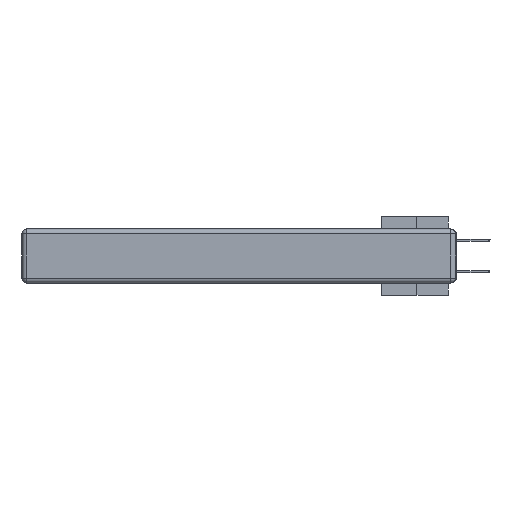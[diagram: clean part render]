
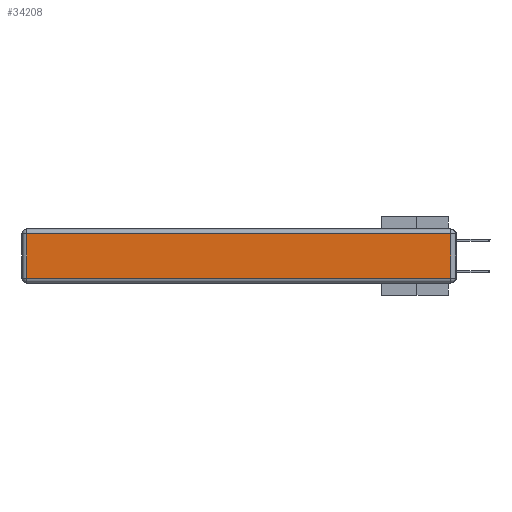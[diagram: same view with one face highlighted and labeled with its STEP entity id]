
A CAD part, left-side view. The second image highlights one B-rep face of the part: STEP entity #34208.
In plain terms, the highlighted planar face has unit normal (-1, 0, 0).
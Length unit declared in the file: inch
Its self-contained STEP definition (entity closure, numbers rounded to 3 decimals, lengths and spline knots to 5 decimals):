
#106 = CARTESIAN_POINT ( 'NONE',  ( 0., 0.03, -0.03 ) ) ;
#294 = CARTESIAN_POINT ( 'NONE',  ( 0., 2.72, -0.313 ) ) ;
#669 = VERTEX_POINT ( 'NONE', #106 ) ;
#1740 = DIRECTION ( 'NONE',  ( 0., -1., 0. ) ) ;
#2527 = DIRECTION ( 'NONE',  ( -1., 0., 0. ) ) ;
#2875 = VECTOR ( 'NONE', #11529, 39.37008 ) ;
#4321 = CARTESIAN_POINT ( 'NONE',  ( 0., 0.03, -0.313 ) ) ;
#6305 = ORIENTED_EDGE ( 'NONE', *, *, #15452, .T. ) ;
#6931 = EDGE_CURVE ( 'NONE', #669, #9083, #14523, .T. ) ;
#8410 = CARTESIAN_POINT ( 'NONE',  ( 0., 0., -0.343 ) ) ;
#8563 = DIRECTION ( 'NONE',  ( 0., 0., 1. ) ) ;
#8766 = PLANE ( 'NONE',  #14390 ) ;
#9083 = VERTEX_POINT ( 'NONE', #27206 ) ;
#9851 = FACE_OUTER_BOUND ( 'NONE', #18857, .T. ) ;
#11529 = DIRECTION ( 'NONE',  ( 0., 0., -1. ) ) ;
#12213 = VERTEX_POINT ( 'NONE', #4321 ) ;
#14390 = AXIS2_PLACEMENT_3D ( 'NONE', #8410, #2527, #31621 ) ;
#14523 = LINE ( 'NONE', #19141, #18632 ) ;
#15293 = LINE ( 'NONE', #17222, #16677 ) ;
#15452 = EDGE_CURVE ( 'NONE', #15798, #12213, #30565, .T. ) ;
#15798 = VERTEX_POINT ( 'NONE', #294 ) ;
#16677 = VECTOR ( 'NONE', #8563, 39.37008 ) ;
#16916 = ORIENTED_EDGE ( 'NONE', *, *, #25487, .T. ) ;
#17143 = CARTESIAN_POINT ( 'NONE',  ( 0., 2.72, -0.343 ) ) ;
#17222 = CARTESIAN_POINT ( 'NONE',  ( 0., 0.03, -0.343 ) ) ;
#17230 = ORIENTED_EDGE ( 'NONE', *, *, #6931, .T. ) ;
#18632 = VECTOR ( 'NONE', #30506, 39.37008 ) ;
#18857 = EDGE_LOOP ( 'NONE', ( #6305, #21646, #17230, #16916 ) ) ;
#19141 = CARTESIAN_POINT ( 'NONE',  ( 0., 2.75, -0.03 ) ) ;
#20972 = VECTOR ( 'NONE', #1740, 39.37008 ) ;
#21646 = ORIENTED_EDGE ( 'NONE', *, *, #24278, .T. ) ;
#24278 = EDGE_CURVE ( 'NONE', #12213, #669, #15293, .T. ) ;
#25487 = EDGE_CURVE ( 'NONE', #9083, #15798, #33013, .T. ) ;
#27206 = CARTESIAN_POINT ( 'NONE',  ( 0., 2.72, -0.03 ) ) ;
#30506 = DIRECTION ( 'NONE',  ( 0., 1., 0. ) ) ;
#30565 = LINE ( 'NONE', #34173, #20972 ) ;
#31621 = DIRECTION ( 'NONE',  ( 0., 0., 1. ) ) ;
#33013 = LINE ( 'NONE', #17143, #2875 ) ;
#34173 = CARTESIAN_POINT ( 'NONE',  ( 0., 0., -0.313 ) ) ;
#34208 = ADVANCED_FACE ( 'NONE', ( #9851 ), #8766, .T. ) ;
